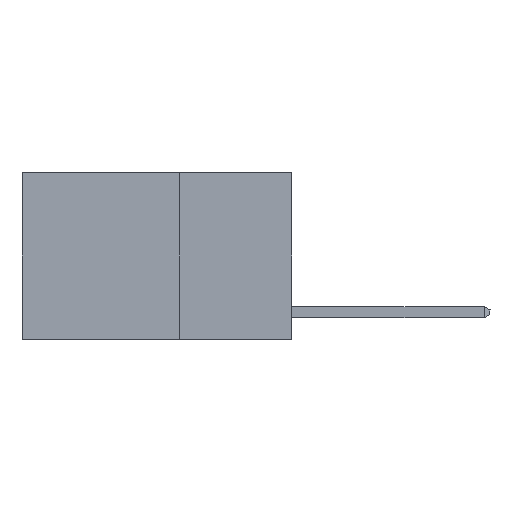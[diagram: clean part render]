
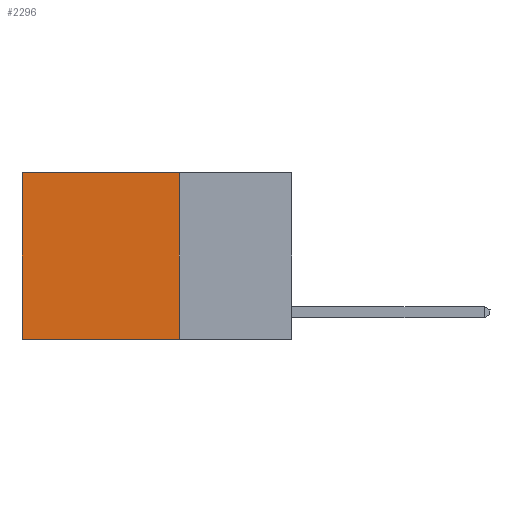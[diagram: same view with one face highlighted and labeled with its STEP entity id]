
A CAD part, left-side view. The second image highlights one B-rep face of the part: STEP entity #2296.
In plain terms, the highlighted planar face has unit normal (-1, 0, 0).
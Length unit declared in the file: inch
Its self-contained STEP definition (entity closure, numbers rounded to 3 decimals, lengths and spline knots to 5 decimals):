
#169 = FACE_OUTER_BOUND ( 'NONE', #10927, .T. ) ;
#334 = EDGE_CURVE ( 'NONE', #9900, #431, #8654, .T. ) ;
#367 = ORIENTED_EDGE ( 'NONE', *, *, #4270, .F. ) ;
#431 = VERTEX_POINT ( 'NONE', #2237 ) ;
#639 = VECTOR ( 'NONE', #6608, 39.37008 ) ;
#769 = EDGE_CURVE ( 'NONE', #431, #3437, #10080, .T. ) ;
#774 = ORIENTED_EDGE ( 'NONE', *, *, #1824, .F. ) ;
#876 = CARTESIAN_POINT ( 'NONE',  ( 0.2625, 0.6, 0. ) ) ;
#1824 = EDGE_CURVE ( 'NONE', #8136, #3437, #2066, .T. ) ;
#2066 = LINE ( 'NONE', #7484, #5133 ) ;
#2237 = CARTESIAN_POINT ( 'NONE',  ( 0.2625, 0.6, 0. ) ) ;
#2296 = ADVANCED_FACE ( 'NONE', ( #169 ), #5344, .F. ) ;
#2814 = AXIS2_PLACEMENT_3D ( 'NONE', #10801, #8223, #11806 ) ;
#3314 = VECTOR ( 'NONE', #5722, 39.37008 ) ;
#3437 = VERTEX_POINT ( 'NONE', #9742 ) ;
#3799 = DIRECTION ( 'NONE',  ( 0., 1., 0. ) ) ;
#3827 = CARTESIAN_POINT ( 'NONE',  ( 0.2625, 0.25, 0. ) ) ;
#4270 = EDGE_CURVE ( 'NONE', #9900, #8136, #6111, .T. ) ;
#5133 = VECTOR ( 'NONE', #3799, 39.37008 ) ;
#5344 = PLANE ( 'NONE',  #2814 ) ;
#5722 = DIRECTION ( 'NONE',  ( 0., 0., -1. ) ) ;
#5750 = CARTESIAN_POINT ( 'NONE',  ( 0.2625, 0.25, 0. ) ) ;
#5770 = CARTESIAN_POINT ( 'NONE',  ( 0.2625, 0.25, 0. ) ) ;
#6111 = LINE ( 'NONE', #3827, #3314 ) ;
#6608 = DIRECTION ( 'NONE',  ( 0., 1., 0. ) ) ;
#7484 = CARTESIAN_POINT ( 'NONE',  ( 0.2625, 0.25, -0.37 ) ) ;
#7856 = ORIENTED_EDGE ( 'NONE', *, *, #769, .T. ) ;
#8136 = VERTEX_POINT ( 'NONE', #11326 ) ;
#8223 = DIRECTION ( 'NONE',  ( 1., 0., 0. ) ) ;
#8362 = DIRECTION ( 'NONE',  ( 0., 0., -1. ) ) ;
#8654 = LINE ( 'NONE', #5770, #639 ) ;
#8749 = ORIENTED_EDGE ( 'NONE', *, *, #334, .T. ) ;
#9742 = CARTESIAN_POINT ( 'NONE',  ( 0.2625, 0.6, -0.37 ) ) ;
#9900 = VERTEX_POINT ( 'NONE', #5750 ) ;
#10080 = LINE ( 'NONE', #876, #11646 ) ;
#10801 = CARTESIAN_POINT ( 'NONE',  ( 0.2625, 0.25, 0. ) ) ;
#10927 = EDGE_LOOP ( 'NONE', ( #7856, #774, #367, #8749 ) ) ;
#11326 = CARTESIAN_POINT ( 'NONE',  ( 0.2625, 0.25, -0.37 ) ) ;
#11646 = VECTOR ( 'NONE', #8362, 39.37008 ) ;
#11806 = DIRECTION ( 'NONE',  ( 0., 0., -1. ) ) ;
